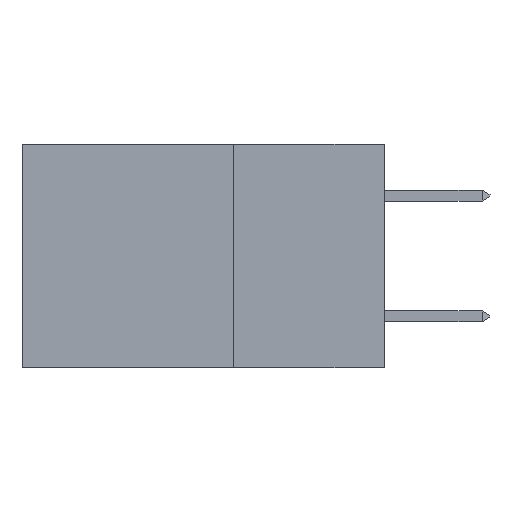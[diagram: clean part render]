
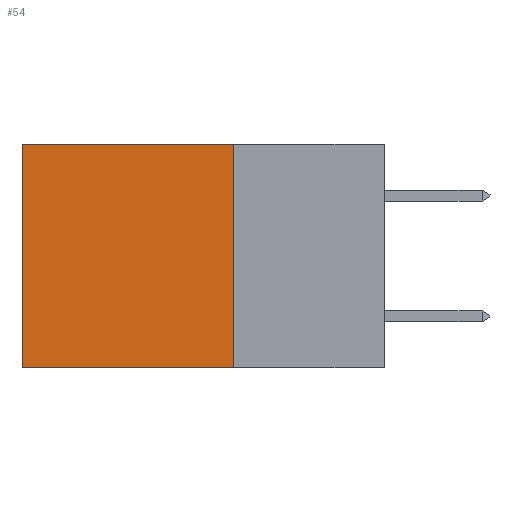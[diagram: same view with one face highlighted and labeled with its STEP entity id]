
A CAD part, left-side view. The second image highlights one B-rep face of the part: STEP entity #54.
In plain terms, the highlighted planar face has unit normal (-1, 0, 0).
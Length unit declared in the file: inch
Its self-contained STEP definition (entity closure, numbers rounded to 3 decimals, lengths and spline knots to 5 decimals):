
#54 = ADVANCED_FACE ( 'NONE', ( #7179 ), #6871, .F. ) ;
#637 = DIRECTION ( 'NONE',  ( 0., 0., -1. ) ) ;
#2676 = VERTEX_POINT ( 'NONE', #14517 ) ;
#4342 = VECTOR ( 'NONE', #637, 39.37008 ) ;
#4912 = EDGE_CURVE ( 'NONE', #10182, #11185, #10797, .T. ) ;
#5146 = CARTESIAN_POINT ( 'NONE',  ( 0.2875, 0.25, -0.37 ) ) ;
#5964 = EDGE_CURVE ( 'NONE', #14162, #2676, #10316, .T. ) ;
#6371 = VECTOR ( 'NONE', #11852, 39.37008 ) ;
#6425 = DIRECTION ( 'NONE',  ( 0., 1., 0. ) ) ;
#6626 = VECTOR ( 'NONE', #6425, 39.37008 ) ;
#6628 = ORIENTED_EDGE ( 'NONE', *, *, #5964, .F. ) ;
#6781 = DIRECTION ( 'NONE',  ( 0., 0., -1. ) ) ;
#6806 = DIRECTION ( 'NONE',  ( 1., 0., 0. ) ) ;
#6871 = PLANE ( 'NONE',  #19679 ) ;
#6928 = LINE ( 'NONE', #21402, #6371 ) ;
#7067 = CARTESIAN_POINT ( 'NONE',  ( 0.2875, 0.25, 0. ) ) ;
#7179 = FACE_OUTER_BOUND ( 'NONE', #15038, .T. ) ;
#7715 = ORIENTED_EDGE ( 'NONE', *, *, #4912, .T. ) ;
#9714 = VECTOR ( 'NONE', #13635, 39.37008 ) ;
#10182 = VERTEX_POINT ( 'NONE', #20984 ) ;
#10316 = LINE ( 'NONE', #12019, #9714 ) ;
#10797 = LINE ( 'NONE', #16482, #6626 ) ;
#10863 = EDGE_CURVE ( 'NONE', #10182, #14162, #21570, .T. ) ;
#11185 = VERTEX_POINT ( 'NONE', #21759 ) ;
#11852 = DIRECTION ( 'NONE',  ( 0., 0., -1. ) ) ;
#12019 = CARTESIAN_POINT ( 'NONE',  ( 0.2875, 0.25, -0.37 ) ) ;
#12949 = CARTESIAN_POINT ( 'NONE',  ( 0.2875, 0.25, 0. ) ) ;
#13412 = ORIENTED_EDGE ( 'NONE', *, *, #20618, .T. ) ;
#13635 = DIRECTION ( 'NONE',  ( 0., 1., 0. ) ) ;
#14162 = VERTEX_POINT ( 'NONE', #5146 ) ;
#14517 = CARTESIAN_POINT ( 'NONE',  ( 0.2875, 0.6, -0.37 ) ) ;
#15038 = EDGE_LOOP ( 'NONE', ( #13412, #6628, #18586, #7715 ) ) ;
#16482 = CARTESIAN_POINT ( 'NONE',  ( 0.2875, 0.25, 0. ) ) ;
#18586 = ORIENTED_EDGE ( 'NONE', *, *, #10863, .F. ) ;
#19679 = AXIS2_PLACEMENT_3D ( 'NONE', #7067, #6806, #6781 ) ;
#20618 = EDGE_CURVE ( 'NONE', #11185, #2676, #6928, .T. ) ;
#20984 = CARTESIAN_POINT ( 'NONE',  ( 0.2875, 0.25, 0. ) ) ;
#21402 = CARTESIAN_POINT ( 'NONE',  ( 0.2875, 0.6, 0. ) ) ;
#21570 = LINE ( 'NONE', #12949, #4342 ) ;
#21759 = CARTESIAN_POINT ( 'NONE',  ( 0.2875, 0.6, 0. ) ) ;
